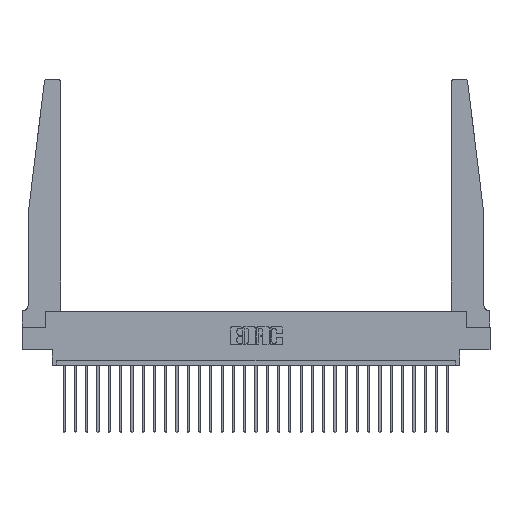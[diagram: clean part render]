
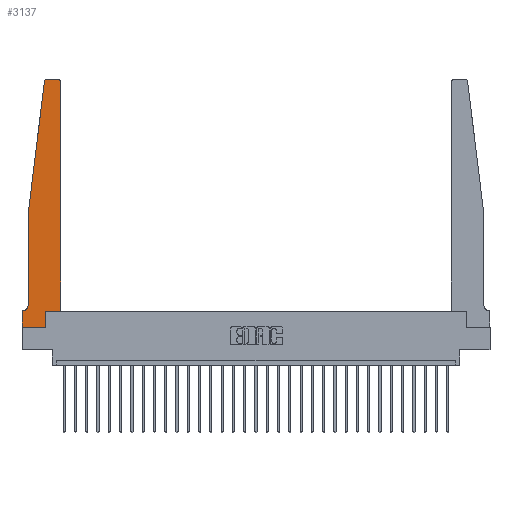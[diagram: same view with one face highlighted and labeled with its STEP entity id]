
A CAD part, top view. The second image highlights one B-rep face of the part: STEP entity #3137.
In plain terms, the highlighted planar face has unit normal (0, 0, 1).
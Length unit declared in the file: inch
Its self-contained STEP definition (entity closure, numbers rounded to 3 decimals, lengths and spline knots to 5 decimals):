
#198 = VECTOR ( 'NONE', #826, 39.37008 ) ;
#358 = EDGE_CURVE ( 'NONE', #15635, #16539, #26644, .T. ) ;
#511 = ORIENTED_EDGE ( 'NONE', *, *, #2995, .T. ) ;
#612 = EDGE_CURVE ( 'NONE', #4209, #20138, #1851, .T. ) ;
#826 = DIRECTION ( 'NONE',  ( 0., 1., 0. ) ) ;
#875 = DIRECTION ( 'NONE',  ( 1., 0., 0. ) ) ;
#1706 = VECTOR ( 'NONE', #2640, 39.37008 ) ;
#1851 = CIRCLE ( 'NONE', #3226, 0.03 ) ;
#2031 = DIRECTION ( 'NONE',  ( -0.122, -0.992, 0. ) ) ;
#2419 = AXIS2_PLACEMENT_3D ( 'NONE', #21594, #18762, #6080 ) ;
#2640 = DIRECTION ( 'NONE',  ( 0., 1., 0. ) ) ;
#2995 = EDGE_CURVE ( 'NONE', #9840, #13624, #15266, .T. ) ;
#3116 = CARTESIAN_POINT ( 'NONE',  ( 0.425, 0.18, 0.37 ) ) ;
#3137 = ADVANCED_FACE ( 'NONE', ( #9569 ), #24739, .T. ) ;
#3226 = AXIS2_PLACEMENT_3D ( 'NONE', #13146, #25894, #19838 ) ;
#3605 = VECTOR ( 'NONE', #875, 39.37008 ) ;
#3615 = VERTEX_POINT ( 'NONE', #12055 ) ;
#3869 = CARTESIAN_POINT ( 'NONE',  ( 0.065, 1.25, 0.37 ) ) ;
#3877 = ORIENTED_EDGE ( 'NONE', *, *, #612, .T. ) ;
#4209 = VERTEX_POINT ( 'NONE', #6995 ) ;
#4864 = EDGE_CURVE ( 'NONE', #19757, #9840, #22858, .T. ) ;
#5055 = EDGE_CURVE ( 'NONE', #10890, #22895, #24157, .T. ) ;
#5764 = EDGE_CURVE ( 'NONE', #20138, #9365, #8556, .T. ) ;
#5773 = CARTESIAN_POINT ( 'NONE',  ( 0.015, 0.1875, 0.37 ) ) ;
#5848 = DIRECTION ( 'NONE',  ( 0., 0., 1. ) ) ;
#5879 = CARTESIAN_POINT ( 'NONE',  ( 0.065, 0.1875, 0.37 ) ) ;
#6080 = DIRECTION ( 'NONE',  ( -1., 0., 0. ) ) ;
#6995 = CARTESIAN_POINT ( 'NONE',  ( 0.27653, 2.75, 0.37 ) ) ;
#7021 = AXIS2_PLACEMENT_3D ( 'NONE', #24890, #5848, #9857 ) ;
#7059 = EDGE_CURVE ( 'NONE', #13935, #4209, #10645, .T. ) ;
#7532 = LINE ( 'NONE', #20889, #13436 ) ;
#7825 = EDGE_LOOP ( 'NONE', ( #16763, #3877, #24215, #16999, #18811, #15090, #15579, #26456, #511, #13983, #10758, #13515 ) ) ;
#8556 = LINE ( 'NONE', #15099, #23267 ) ;
#8748 = VECTOR ( 'NONE', #14939, 39.37008 ) ;
#9365 = VERTEX_POINT ( 'NONE', #3869 ) ;
#9569 = FACE_OUTER_BOUND ( 'NONE', #7825, .T. ) ;
#9782 = CARTESIAN_POINT ( 'NONE',  ( 0.425, 2.72, 0.37 ) ) ;
#9840 = VERTEX_POINT ( 'NONE', #27769 ) ;
#9857 = DIRECTION ( 'NONE',  ( 1., 0., 0. ) ) ;
#10645 = LINE ( 'NONE', #19335, #8748 ) ;
#10758 = ORIENTED_EDGE ( 'NONE', *, *, #358, .T. ) ;
#10890 = VERTEX_POINT ( 'NONE', #14415 ) ;
#12037 = LINE ( 'NONE', #24429, #15476 ) ;
#12055 = CARTESIAN_POINT ( 'NONE',  ( 0., 0.1875, 0.37 ) ) ;
#12204 = CARTESIAN_POINT ( 'NONE',  ( 0., 0., 0.37 ) ) ;
#13117 = CARTESIAN_POINT ( 'NONE',  ( 0.2605, 0.18, 0.37 ) ) ;
#13146 = CARTESIAN_POINT ( 'NONE',  ( 0.27653, 2.72, 0.37 ) ) ;
#13436 = VECTOR ( 'NONE', #16235, 39.37008 ) ;
#13515 = ORIENTED_EDGE ( 'NONE', *, *, #18820, .T. ) ;
#13624 = VERTEX_POINT ( 'NONE', #18570 ) ;
#13815 = DIRECTION ( 'NONE',  ( 0., 0., 1. ) ) ;
#13935 = VERTEX_POINT ( 'NONE', #26852 ) ;
#13983 = ORIENTED_EDGE ( 'NONE', *, *, #17662, .T. ) ;
#14415 = CARTESIAN_POINT ( 'NONE',  ( 0.065, 0.2375, 0.37 ) ) ;
#14458 = VECTOR ( 'NONE', #23208, 39.37008 ) ;
#14714 = LINE ( 'NONE', #5879, #14458 ) ;
#14939 = DIRECTION ( 'NONE',  ( -1., 0., 0. ) ) ;
#15090 = ORIENTED_EDGE ( 'NONE', *, *, #24661, .T. ) ;
#15099 = CARTESIAN_POINT ( 'NONE',  ( 0.065, 1.25, 0.37 ) ) ;
#15266 = LINE ( 'NONE', #13117, #1706 ) ;
#15476 = VECTOR ( 'NONE', #26664, 39.37008 ) ;
#15579 = ORIENTED_EDGE ( 'NONE', *, *, #20551, .T. ) ;
#15635 = VERTEX_POINT ( 'NONE', #18122 ) ;
#16120 = DIRECTION ( 'NONE',  ( 1., 0., 0. ) ) ;
#16235 = DIRECTION ( 'NONE',  ( 0., -1., 0. ) ) ;
#16539 = VERTEX_POINT ( 'NONE', #9782 ) ;
#16763 = ORIENTED_EDGE ( 'NONE', *, *, #7059, .T. ) ;
#16999 = ORIENTED_EDGE ( 'NONE', *, *, #18618, .T. ) ;
#17275 = CARTESIAN_POINT ( 'NONE',  ( 0., 0., 0.37 ) ) ;
#17507 = CIRCLE ( 'NONE', #7021, 0.03 ) ;
#17662 = EDGE_CURVE ( 'NONE', #13624, #15635, #12037, .T. ) ;
#17985 = LINE ( 'NONE', #24063, #21114 ) ;
#18122 = CARTESIAN_POINT ( 'NONE',  ( 0.425, 0.18, 0.37 ) ) ;
#18570 = CARTESIAN_POINT ( 'NONE',  ( 0.2605, 0.18, 0.37 ) ) ;
#18618 = EDGE_CURVE ( 'NONE', #9365, #10890, #17985, .T. ) ;
#18762 = DIRECTION ( 'NONE',  ( 0., 0., -1. ) ) ;
#18811 = ORIENTED_EDGE ( 'NONE', *, *, #5055, .T. ) ;
#18820 = EDGE_CURVE ( 'NONE', #16539, #13935, #17507, .T. ) ;
#19335 = CARTESIAN_POINT ( 'NONE',  ( 0.25, 2.75, 0.37 ) ) ;
#19757 = VERTEX_POINT ( 'NONE', #17275 ) ;
#19838 = DIRECTION ( 'NONE',  ( 1., 0., 0. ) ) ;
#20138 = VERTEX_POINT ( 'NONE', #23324 ) ;
#20551 = EDGE_CURVE ( 'NONE', #3615, #19757, #7532, .T. ) ;
#20889 = CARTESIAN_POINT ( 'NONE',  ( 0., 0., 0.37 ) ) ;
#21114 = VECTOR ( 'NONE', #24208, 39.37008 ) ;
#21594 = CARTESIAN_POINT ( 'NONE',  ( 0.015, 0.2375, 0.37 ) ) ;
#22858 = LINE ( 'NONE', #12204, #3605 ) ;
#22895 = VERTEX_POINT ( 'NONE', #5773 ) ;
#23208 = DIRECTION ( 'NONE',  ( -1., 0., 0. ) ) ;
#23267 = VECTOR ( 'NONE', #2031, 39.37008 ) ;
#23324 = CARTESIAN_POINT ( 'NONE',  ( 0.24675, 2.72367, 0.37 ) ) ;
#24063 = CARTESIAN_POINT ( 'NONE',  ( 0.065, 1.25, 0.37 ) ) ;
#24157 = CIRCLE ( 'NONE', #2419, 0.05 ) ;
#24208 = DIRECTION ( 'NONE',  ( 0., -1., 0. ) ) ;
#24215 = ORIENTED_EDGE ( 'NONE', *, *, #5764, .T. ) ;
#24369 = AXIS2_PLACEMENT_3D ( 'NONE', #27247, #13815, #16120 ) ;
#24429 = CARTESIAN_POINT ( 'NONE',  ( 0.425, 0.18, 0.37 ) ) ;
#24661 = EDGE_CURVE ( 'NONE', #22895, #3615, #14714, .T. ) ;
#24739 = PLANE ( 'NONE',  #24369 ) ;
#24890 = CARTESIAN_POINT ( 'NONE',  ( 0.395, 2.72, 0.37 ) ) ;
#25894 = DIRECTION ( 'NONE',  ( 0., 0., 1. ) ) ;
#26456 = ORIENTED_EDGE ( 'NONE', *, *, #4864, .T. ) ;
#26644 = LINE ( 'NONE', #3116, #198 ) ;
#26664 = DIRECTION ( 'NONE',  ( 1., 0., 0. ) ) ;
#26852 = CARTESIAN_POINT ( 'NONE',  ( 0.395, 2.75, 0.37 ) ) ;
#27247 = CARTESIAN_POINT ( 'NONE',  ( 0., 0.1875, 0.37 ) ) ;
#27769 = CARTESIAN_POINT ( 'NONE',  ( 0.2605, 0., 0.37 ) ) ;
